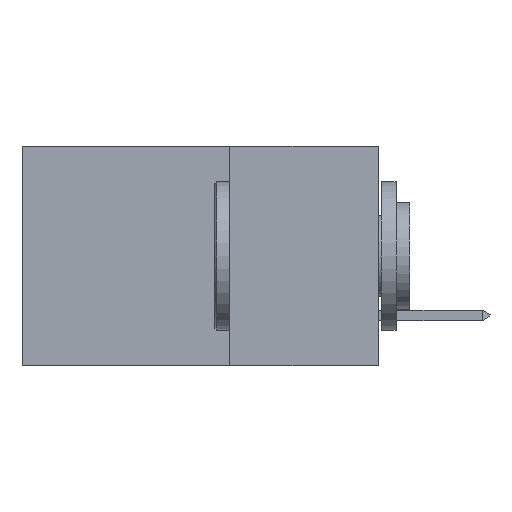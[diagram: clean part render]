
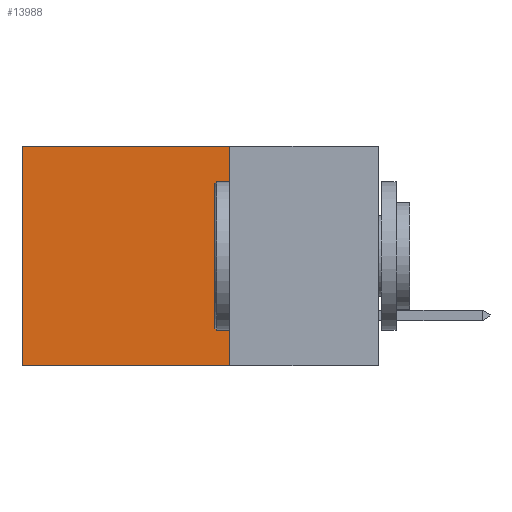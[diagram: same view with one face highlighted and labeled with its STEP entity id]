
A CAD part, left-side view. The second image highlights one B-rep face of the part: STEP entity #13988.
In plain terms, the highlighted planar face has unit normal (-1, 0, 0).
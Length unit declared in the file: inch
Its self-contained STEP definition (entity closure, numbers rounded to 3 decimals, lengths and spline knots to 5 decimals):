
#400 = DIRECTION ( 'NONE',  ( 0., 0., -1. ) ) ;
#690 = CARTESIAN_POINT ( 'NONE',  ( 0.298, 0.25, 0. ) ) ;
#833 = DIRECTION ( 'NONE',  ( 0., 0., -1. ) ) ;
#1285 = CARTESIAN_POINT ( 'NONE',  ( 0.298, 0.6, -0.37 ) ) ;
#2344 = VERTEX_POINT ( 'NONE', #8276 ) ;
#3186 = ORIENTED_EDGE ( 'NONE', *, *, #27157, .T. ) ;
#3947 = PLANE ( 'NONE',  #9123 ) ;
#5243 = LINE ( 'NONE', #26195, #16863 ) ;
#5909 = EDGE_CURVE ( 'NONE', #17655, #27762, #5243, .T. ) ;
#7209 = DIRECTION ( 'NONE',  ( 0., 1., 0. ) ) ;
#7315 = CARTESIAN_POINT ( 'NONE',  ( 0.298, 0.6, 0. ) ) ;
#8276 = CARTESIAN_POINT ( 'NONE',  ( 0.298, 0.6, 0. ) ) ;
#8319 = ORIENTED_EDGE ( 'NONE', *, *, #21477, .F. ) ;
#8702 = LINE ( 'NONE', #7315, #18995 ) ;
#9123 = AXIS2_PLACEMENT_3D ( 'NONE', #17224, #21457, #23660 ) ;
#10485 = EDGE_LOOP ( 'NONE', ( #3186, #8319, #21483, #16794 ) ) ;
#13159 = VECTOR ( 'NONE', #19075, 39.37008 ) ;
#13988 = ADVANCED_FACE ( 'NONE', ( #17997 ), #3947, .F. ) ;
#14641 = EDGE_CURVE ( 'NONE', #17655, #2344, #24798, .T. ) ;
#14673 = VERTEX_POINT ( 'NONE', #1285 ) ;
#16794 = ORIENTED_EDGE ( 'NONE', *, *, #14641, .T. ) ;
#16863 = VECTOR ( 'NONE', #400, 39.37008 ) ;
#17224 = CARTESIAN_POINT ( 'NONE',  ( 0.298, 0.25, 0. ) ) ;
#17655 = VERTEX_POINT ( 'NONE', #690 ) ;
#17997 = FACE_OUTER_BOUND ( 'NONE', #10485, .T. ) ;
#18681 = VECTOR ( 'NONE', #7209, 39.37008 ) ;
#18995 = VECTOR ( 'NONE', #833, 39.37008 ) ;
#19075 = DIRECTION ( 'NONE',  ( 0., 1., 0. ) ) ;
#21457 = DIRECTION ( 'NONE',  ( 1., 0., 0. ) ) ;
#21477 = EDGE_CURVE ( 'NONE', #27762, #14673, #23827, .T. ) ;
#21483 = ORIENTED_EDGE ( 'NONE', *, *, #5909, .F. ) ;
#22604 = CARTESIAN_POINT ( 'NONE',  ( 0.298, 0.25, 0. ) ) ;
#23660 = DIRECTION ( 'NONE',  ( 0., 0., -1. ) ) ;
#23827 = LINE ( 'NONE', #26628, #18681 ) ;
#24798 = LINE ( 'NONE', #22604, #13159 ) ;
#26195 = CARTESIAN_POINT ( 'NONE',  ( 0.298, 0.25, 0. ) ) ;
#26628 = CARTESIAN_POINT ( 'NONE',  ( 0.298, 0.25, -0.37 ) ) ;
#27157 = EDGE_CURVE ( 'NONE', #2344, #14673, #8702, .T. ) ;
#27762 = VERTEX_POINT ( 'NONE', #27805 ) ;
#27805 = CARTESIAN_POINT ( 'NONE',  ( 0.298, 0.25, -0.37 ) ) ;
